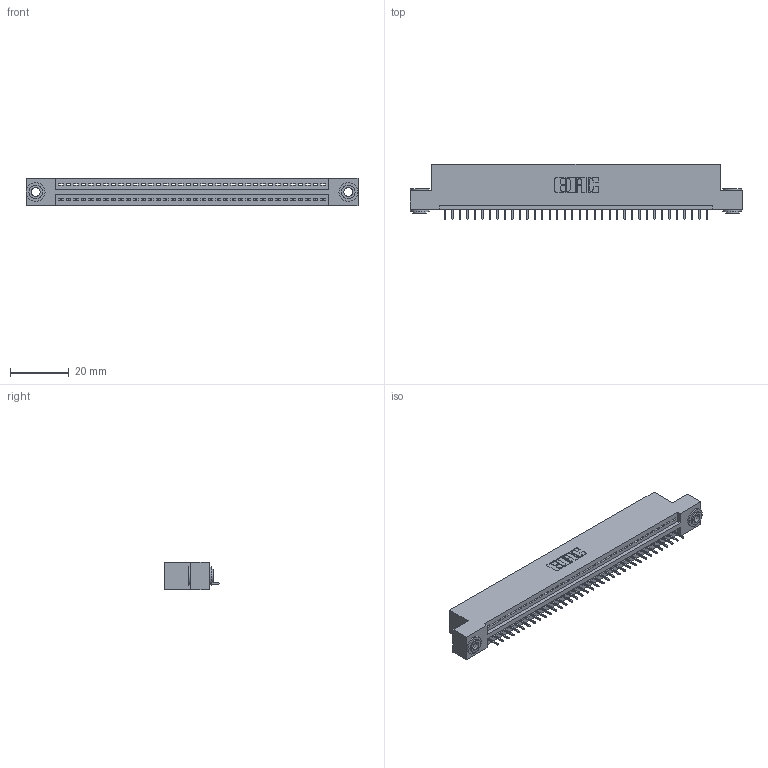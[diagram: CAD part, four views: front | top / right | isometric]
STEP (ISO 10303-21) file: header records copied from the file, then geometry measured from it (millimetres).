
FILE_DESCRIPTION (( 'STEP AP203' ), '1' );
FILE_NAME ('845-036-525-103.STEP', '2020-09-23T02:45:36', ( '' ), ( '' ), 'SwSTEP 2.0', 'SolidWorks 2020', '' );
FILE_SCHEMA (( 'CONFIG_CONTROL_DESIGN' ));
Length unit declared in the file: inch
Products named in the file (4): 345-250-002_345-250-002-102; 345-292-001_345-293-125; 845 Part_Flush Mounting Lugs - 0.156 Dia-TH; 845-036-525-103
Assembly tree (39 placements, depth 2):
  845-036-525-103
    845 Part_Flush Mounting Lugs - 0.156 Dia-TH
    345-292-001_345-293-125  x36
    345-250-002_345-250-002-102  x2
Bounding box: 112.65 x 18.72 x 9.4 mm (x, y, z)
Volume: 10522.8 mm3; surface area: 13626.6 mm2
Topology: 39 solids, 39 shells, 2396 faces, 6897 edges, 4450 vertices
Faces by surface type: plane 1746, cylinder 642, cone 8
Entity records: 28626 total; most frequent: CARTESIAN_POINT 4935, ORIENTED_EDGE 4898, DIRECTION 4351, EDGE_CURVE 2449, VECTOR 2153, LINE 2153, VERTEX_POINT 1626, AXIS2_PLACEMENT_3D 1099
